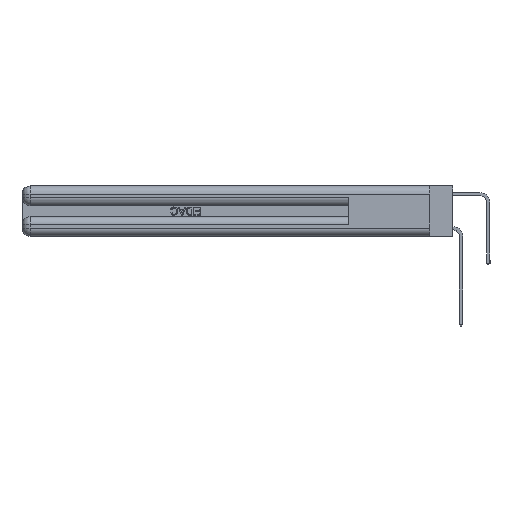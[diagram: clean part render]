
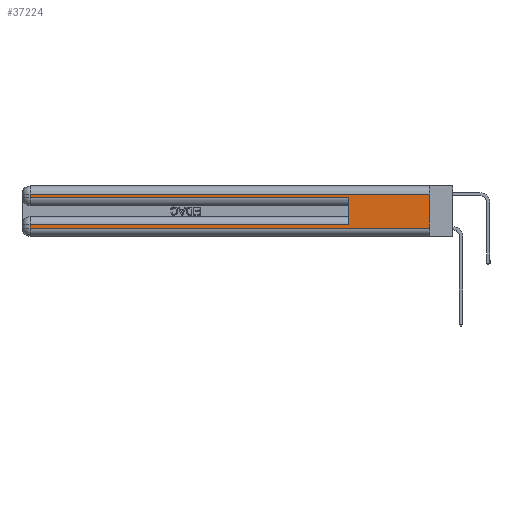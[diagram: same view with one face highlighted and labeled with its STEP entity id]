
A CAD part, left-side view. The second image highlights one B-rep face of the part: STEP entity #37224.
In plain terms, the highlighted planar face has unit normal (-1, 0, 0).
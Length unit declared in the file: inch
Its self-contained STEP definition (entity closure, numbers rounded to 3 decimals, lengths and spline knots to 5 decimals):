
#1069 = DIRECTION ( 'NONE',  ( 0., 0., -1. ) ) ;
#1693 = CARTESIAN_POINT ( 'NONE',  ( 0., 0., 0.31 ) ) ;
#1847 = VECTOR ( 'NONE', #23545, 39.37008 ) ;
#2553 = AXIS2_PLACEMENT_3D ( 'NONE', #27125, #26395, #1069 ) ;
#2690 = CARTESIAN_POINT ( 'NONE',  ( 0., 0., 0.37 ) ) ;
#2701 = VERTEX_POINT ( 'NONE', #28996 ) ;
#3125 = VERTEX_POINT ( 'NONE', #4042 ) ;
#4042 = CARTESIAN_POINT ( 'NONE',  ( 0., 0., 0.31 ) ) ;
#5355 = EDGE_CURVE ( 'NONE', #17041, #16757, #16502, .T. ) ;
#5653 = CARTESIAN_POINT ( 'NONE',  ( 0., 2.94, 0.37 ) ) ;
#5975 = ORIENTED_EDGE ( 'NONE', *, *, #5355, .T. ) ;
#6121 = CARTESIAN_POINT ( 'NONE',  ( 0., 2.94, 0.085 ) ) ;
#6441 = ORIENTED_EDGE ( 'NONE', *, *, #29377, .T. ) ;
#6468 = EDGE_CURVE ( 'NONE', #14088, #2701, #35953, .T. ) ;
#6835 = VERTEX_POINT ( 'NONE', #29786 ) ;
#7531 = CARTESIAN_POINT ( 'NONE',  ( 0., 0., 0.06 ) ) ;
#7553 = VERTEX_POINT ( 'NONE', #15592 ) ;
#8061 = ORIENTED_EDGE ( 'NONE', *, *, #14410, .F. ) ;
#8600 = DIRECTION ( 'NONE',  ( 0., 0., -1. ) ) ;
#9075 = ORIENTED_EDGE ( 'NONE', *, *, #12748, .T. ) ;
#12748 = EDGE_CURVE ( 'NONE', #3125, #31361, #30431, .T. ) ;
#13825 = VECTOR ( 'NONE', #21698, 39.37008 ) ;
#14088 = VERTEX_POINT ( 'NONE', #19969 ) ;
#14410 = EDGE_CURVE ( 'NONE', #6835, #2701, #28278, .T. ) ;
#14980 = FACE_OUTER_BOUND ( 'NONE', #18283, .T. ) ;
#15315 = VECTOR ( 'NONE', #16120, 39.37008 ) ;
#15502 = EDGE_CURVE ( 'NONE', #3125, #7553, #28193, .T. ) ;
#15592 = CARTESIAN_POINT ( 'NONE',  ( 0., 0., 0.06 ) ) ;
#16079 = ORIENTED_EDGE ( 'NONE', *, *, #6468, .T. ) ;
#16120 = DIRECTION ( 'NONE',  ( 0., 0., 1. ) ) ;
#16502 = LINE ( 'NONE', #5653, #18576 ) ;
#16561 = VECTOR ( 'NONE', #33775, 39.37008 ) ;
#16608 = CARTESIAN_POINT ( 'NONE',  ( 0., 2.94, 0.06 ) ) ;
#16757 = VERTEX_POINT ( 'NONE', #16608 ) ;
#17041 = VERTEX_POINT ( 'NONE', #6121 ) ;
#18283 = EDGE_LOOP ( 'NONE', ( #36817, #9075, #6441, #16079, #8061, #23433, #5975, #19359 ) ) ;
#18576 = VECTOR ( 'NONE', #37225, 39.37008 ) ;
#18979 = CARTESIAN_POINT ( 'NONE',  ( 0., 0.6, 0.145 ) ) ;
#19359 = ORIENTED_EDGE ( 'NONE', *, *, #20558, .T. ) ;
#19969 = CARTESIAN_POINT ( 'NONE',  ( 0., 2.94, 0.285 ) ) ;
#20558 = EDGE_CURVE ( 'NONE', #16757, #7553, #22179, .T. ) ;
#20870 = VECTOR ( 'NONE', #8600, 39.37008 ) ;
#21698 = DIRECTION ( 'NONE',  ( 0., -1., 0. ) ) ;
#22179 = LINE ( 'NONE', #7531, #16561 ) ;
#22611 = DIRECTION ( 'NONE',  ( 0., 1., 0. ) ) ;
#23091 = LINE ( 'NONE', #34687, #36485 ) ;
#23433 = ORIENTED_EDGE ( 'NONE', *, *, #31571, .T. ) ;
#23545 = DIRECTION ( 'NONE',  ( 0., 0., -1. ) ) ;
#25198 = CARTESIAN_POINT ( 'NONE',  ( 0., 2.94, 0.31 ) ) ;
#26395 = DIRECTION ( 'NONE',  ( 1., 0., 0. ) ) ;
#26576 = CARTESIAN_POINT ( 'NONE',  ( 0., 2.94, 0.37 ) ) ;
#27125 = CARTESIAN_POINT ( 'NONE',  ( 0., 0., 0.37 ) ) ;
#28193 = LINE ( 'NONE', #2690, #20870 ) ;
#28278 = LINE ( 'NONE', #18979, #15315 ) ;
#28996 = CARTESIAN_POINT ( 'NONE',  ( 0., 0.6, 0.285 ) ) ;
#29377 = EDGE_CURVE ( 'NONE', #31361, #14088, #34955, .T. ) ;
#29622 = PLANE ( 'NONE',  #2553 ) ;
#29786 = CARTESIAN_POINT ( 'NONE',  ( 0., 0.6, 0.085 ) ) ;
#29879 = CARTESIAN_POINT ( 'NONE',  ( 0., 0., 0.285 ) ) ;
#30431 = LINE ( 'NONE', #1693, #35427 ) ;
#31361 = VERTEX_POINT ( 'NONE', #25198 ) ;
#31571 = EDGE_CURVE ( 'NONE', #6835, #17041, #23091, .T. ) ;
#33775 = DIRECTION ( 'NONE',  ( 0., -1., 0. ) ) ;
#34224 = DIRECTION ( 'NONE',  ( 0., 1., 0. ) ) ;
#34687 = CARTESIAN_POINT ( 'NONE',  ( 0., 0., 0.085 ) ) ;
#34955 = LINE ( 'NONE', #26576, #1847 ) ;
#35427 = VECTOR ( 'NONE', #34224, 39.37008 ) ;
#35953 = LINE ( 'NONE', #29879, #13825 ) ;
#36485 = VECTOR ( 'NONE', #22611, 39.37008 ) ;
#36817 = ORIENTED_EDGE ( 'NONE', *, *, #15502, .F. ) ;
#37224 = ADVANCED_FACE ( 'NONE', ( #14980 ), #29622, .F. ) ;
#37225 = DIRECTION ( 'NONE',  ( 0., 0., -1. ) ) ;
